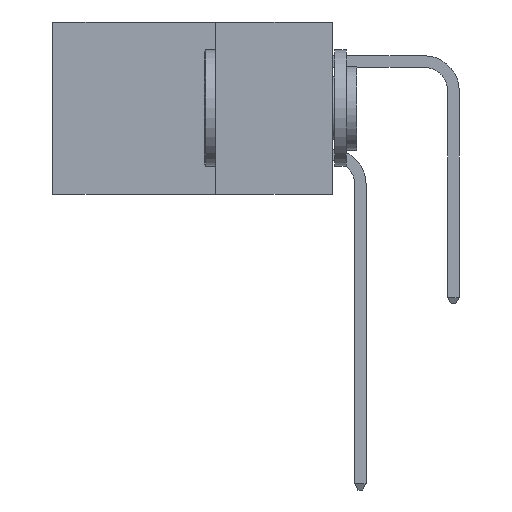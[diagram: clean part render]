
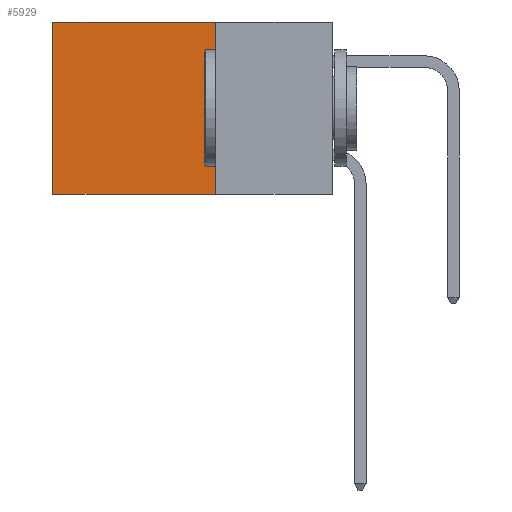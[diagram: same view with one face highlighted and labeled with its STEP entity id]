
A CAD part, left-side view. The second image highlights one B-rep face of the part: STEP entity #5929.
In plain terms, the highlighted planar face has unit normal (-1, 0, 0).
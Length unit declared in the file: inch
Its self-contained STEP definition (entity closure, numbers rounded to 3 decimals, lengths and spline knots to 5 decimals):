
#282 = LINE ( 'NONE', #8758, #4060 ) ;
#1266 = CARTESIAN_POINT ( 'NONE',  ( 0.2615, 0.6, -0.37 ) ) ;
#1787 = CARTESIAN_POINT ( 'NONE',  ( 0.2615, 0.25, 0. ) ) ;
#3276 = AXIS2_PLACEMENT_3D ( 'NONE', #11387, #4639, #12447 ) ;
#3841 = ORIENTED_EDGE ( 'NONE', *, *, #5856, .T. ) ;
#3973 = DIRECTION ( 'NONE',  ( 0., 1., 0. ) ) ;
#4060 = VECTOR ( 'NONE', #3973, 39.37008 ) ;
#4639 = DIRECTION ( 'NONE',  ( 1., 0., 0. ) ) ;
#4737 = FACE_OUTER_BOUND ( 'NONE', #4870, .T. ) ;
#4870 = EDGE_LOOP ( 'NONE', ( #3841, #10814, #11427, #11216 ) ) ;
#5044 = VECTOR ( 'NONE', #7991, 39.37008 ) ;
#5207 = LINE ( 'NONE', #7159, #7670 ) ;
#5322 = CARTESIAN_POINT ( 'NONE',  ( 0.2615, 0.6, -0.37 ) ) ;
#5578 = EDGE_CURVE ( 'NONE', #7302, #7327, #5207, .T. ) ;
#5856 = EDGE_CURVE ( 'NONE', #7327, #7643, #7018, .T. ) ;
#5929 = ADVANCED_FACE ( 'NONE', ( #4737 ), #11517, .F. ) ;
#5957 = VERTEX_POINT ( 'NONE', #7547 ) ;
#7018 = LINE ( 'NONE', #1266, #5044 ) ;
#7029 = DIRECTION ( 'NONE',  ( 0., 1., 0. ) ) ;
#7159 = CARTESIAN_POINT ( 'NONE',  ( 0.2615, 0.25, 0. ) ) ;
#7302 = VERTEX_POINT ( 'NONE', #1787 ) ;
#7327 = VERTEX_POINT ( 'NONE', #8493 ) ;
#7547 = CARTESIAN_POINT ( 'NONE',  ( 0.2615, 0.25, -0.37 ) ) ;
#7643 = VERTEX_POINT ( 'NONE', #5322 ) ;
#7670 = VECTOR ( 'NONE', #7029, 39.37008 ) ;
#7991 = DIRECTION ( 'NONE',  ( 0., 0., -1. ) ) ;
#8493 = CARTESIAN_POINT ( 'NONE',  ( 0.2615, 0.6, 0. ) ) ;
#8758 = CARTESIAN_POINT ( 'NONE',  ( 0.2615, 0.25, -0.37 ) ) ;
#9531 = CARTESIAN_POINT ( 'NONE',  ( 0.2615, 0.25, -0.37 ) ) ;
#9777 = EDGE_CURVE ( 'NONE', #5957, #7643, #282, .T. ) ;
#10313 = LINE ( 'NONE', #9531, #12252 ) ;
#10814 = ORIENTED_EDGE ( 'NONE', *, *, #9777, .F. ) ;
#11109 = EDGE_CURVE ( 'NONE', #7302, #5957, #10313, .T. ) ;
#11216 = ORIENTED_EDGE ( 'NONE', *, *, #5578, .T. ) ;
#11387 = CARTESIAN_POINT ( 'NONE',  ( 0.2615, 0.25, -0.37 ) ) ;
#11427 = ORIENTED_EDGE ( 'NONE', *, *, #11109, .F. ) ;
#11494 = DIRECTION ( 'NONE',  ( 0., 0., -1. ) ) ;
#11517 = PLANE ( 'NONE',  #3276 ) ;
#12252 = VECTOR ( 'NONE', #11494, 39.37008 ) ;
#12447 = DIRECTION ( 'NONE',  ( 0., 0., -1. ) ) ;
